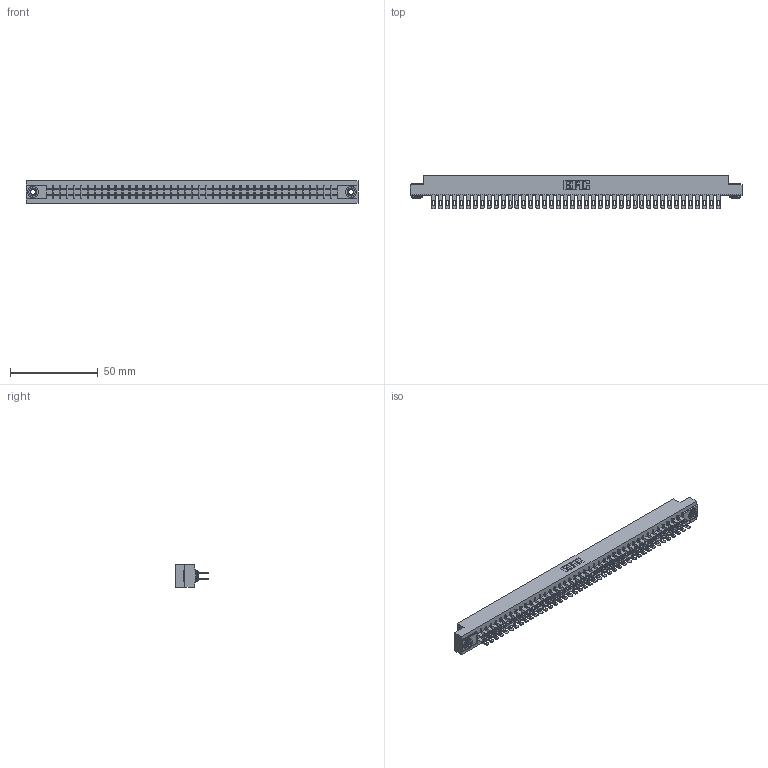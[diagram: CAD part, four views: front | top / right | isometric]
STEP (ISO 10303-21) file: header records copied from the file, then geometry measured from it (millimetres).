
FILE_DESCRIPTION (( 'STEP AP203' ), '1' );
FILE_NAME ('355-084-500-503.STEP', '2019-09-13T15:44:05', ( '' ), ( '' ), 'SwSTEP 2.0', 'SolidWorks 2016', '' );
FILE_SCHEMA (( 'CONFIG_CONTROL_DESIGN' ));
Length unit declared in the file: inch
Products named in the file (4): 355-084-500-503; 305-290-001_500; 305 Part_.156 Dia; 345-250-002_345-250-002-102
Assembly tree (87 placements, depth 2):
  355-084-500-503
    305 Part_.156 Dia
    305-290-001_500  x84
    345-250-002_345-250-002-102  x2
Bounding box: 189.43 x 18.85 x 12.7 mm (x, y, z)
Volume: 19442.9 mm3; surface area: 27560 mm2
Topology: 87 solids, 87 shells, 4368 faces, 12482 edges, 8092 vertices
Faces by surface type: plane 2444, cylinder 1748, sphere 168, cone 8
Entity records: 46562 total; most frequent: CARTESIAN_POINT 7685, ORIENTED_EDGE 7620, DIRECTION 7452, EDGE_CURVE 3810, LINE 3070, VECTOR 3070, VERTEX_POINT 2424, AXIS2_PLACEMENT_3D 2191
